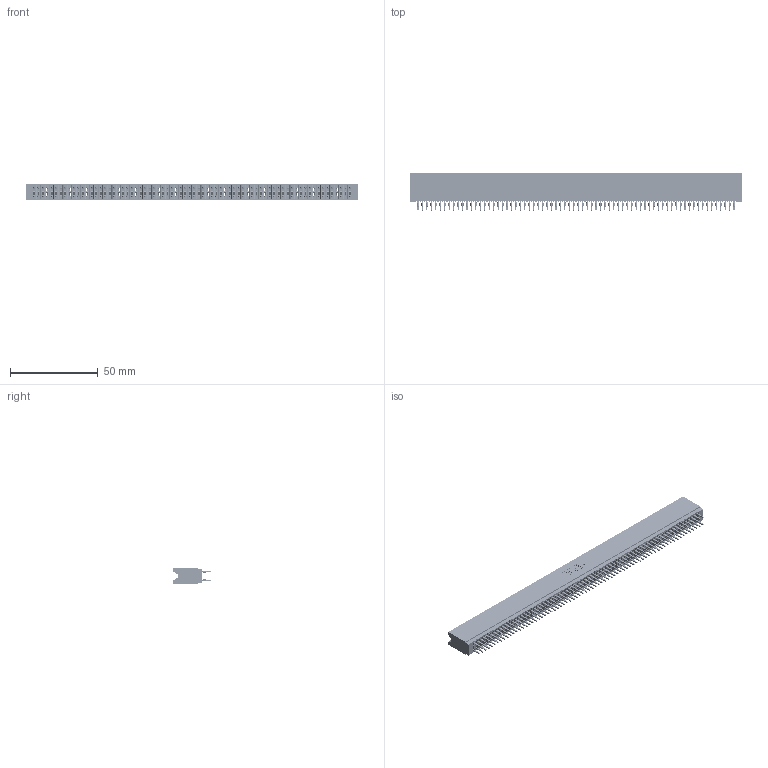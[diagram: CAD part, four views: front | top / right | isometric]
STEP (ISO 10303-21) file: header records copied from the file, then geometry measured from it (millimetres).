
FILE_DESCRIPTION (( 'STEP AP203' ), '1' );
FILE_NAME ('745-144-560-206.STEP', '2026-02-27T04:24:40', ( '' ), ( '' ), 'SwSTEP 2.0', 'SolidWorks 2023', '' );
FILE_SCHEMA (( 'CONFIG_CONTROL_DESIGN' ));
Length unit declared in the file: millimetre
Products named in the file (3): 745 Part_Insulator Option - 06; 745-144-560-206; 745-292-001_560
Assembly tree (145 placements, depth 2):
  745-144-560-206
    745 Part_Insulator Option - 06
    745-292-001_560  x144
Bounding box: 189.48 x 21.22 x 8.89 mm (x, y, z)
Volume: 17393.2 mm3; surface area: 38352.3 mm2
Topology: 145 solids, 145 shells, 14280 faces, 39068 edges, 24796 vertices
Faces by surface type: plane 7400, cylinder 3136, bspline 2880, torus 864
Entity records: 117461 total; most frequent: CARTESIAN_POINT 20868, ORIENTED_EDGE 20364, DIRECTION 17768, EDGE_CURVE 10182, LINE 9560, VECTOR 9560, VERTEX_POINT 6492, AXIS2_PLACEMENT_3D 4104
